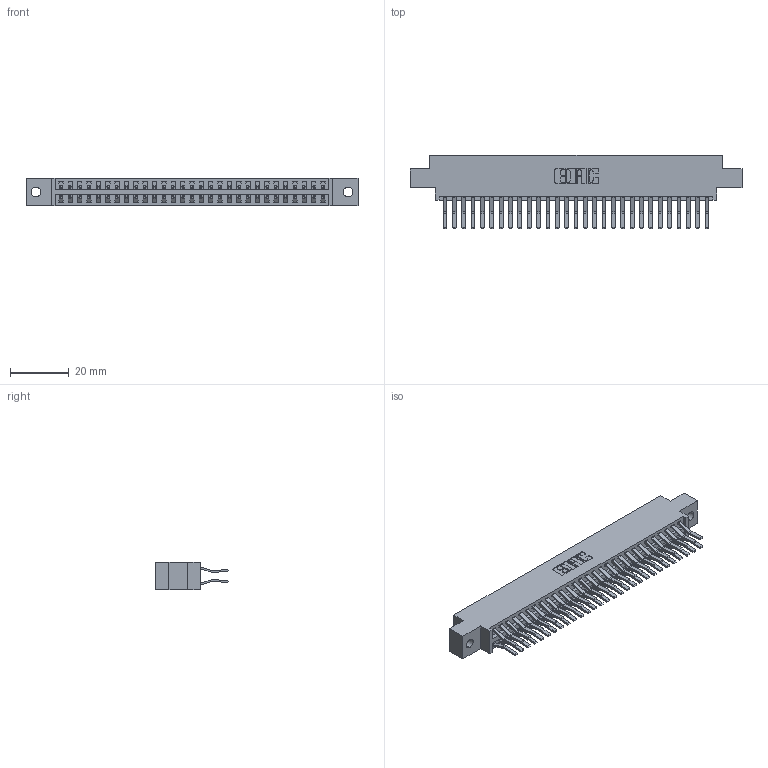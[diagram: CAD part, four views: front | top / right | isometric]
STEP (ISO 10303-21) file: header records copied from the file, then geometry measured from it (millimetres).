
FILE_DESCRIPTION (( 'STEP AP203' ), '1' );
FILE_NAME ('346-058-560-802.STEP', '2018-08-28T05:00:30', ( '' ), ( '' ), 'SwSTEP 2.0', 'SolidWorks 2016', '' );
FILE_SCHEMA (( 'CONFIG_CONTROL_DESIGN' ));
Length unit declared in the file: inch
Products named in the file (3): 346 Part_0.170 Offset - 0.128 Dia; 345-292-001_560 Tail; 346-058-560-802
Assembly tree (59 placements, depth 2):
  346-058-560-802
    346 Part_0.170 Offset - 0.128 Dia
    345-292-001_560 Tail  x58
Bounding box: 112.65 x 24.78 x 9.4 mm (x, y, z)
Volume: 11072.6 mm3; surface area: 15940.3 mm2
Topology: 59 solids, 59 shells, 3258 faces, 9679 edges, 6374 vertices
Faces by surface type: plane 2110, cylinder 1148
Entity records: 20899 total; most frequent: CARTESIAN_POINT 3464, ORIENTED_EDGE 3398, DIRECTION 3107, EDGE_CURVE 1699, LINE 1447, VECTOR 1447, VERTEX_POINT 1130, AXIS2_PLACEMENT_3D 830
